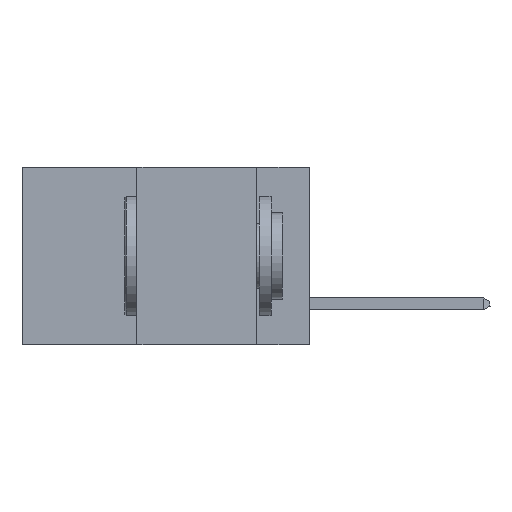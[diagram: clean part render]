
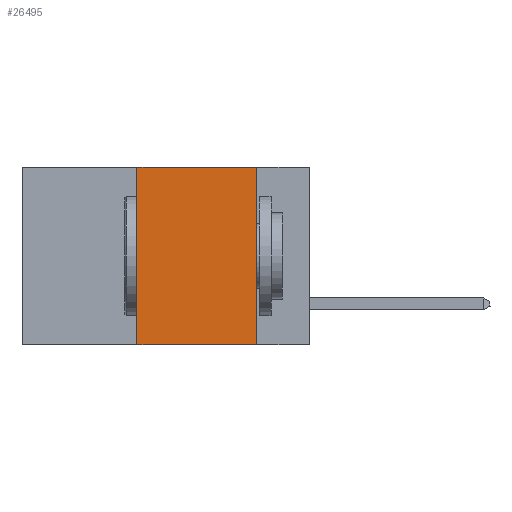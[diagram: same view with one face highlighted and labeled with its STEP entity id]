
A CAD part, left-side view. The second image highlights one B-rep face of the part: STEP entity #26495.
In plain terms, the highlighted planar face has unit normal (-1, 0, 0).
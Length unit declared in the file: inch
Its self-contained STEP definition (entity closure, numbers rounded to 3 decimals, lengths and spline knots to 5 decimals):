
#259 = EDGE_CURVE ( 'NONE', #32341, #35100, #21879, .T. ) ;
#385 = CARTESIAN_POINT ( 'NONE',  ( 0., 0.6, -0.37 ) ) ;
#1940 = AXIS2_PLACEMENT_3D ( 'NONE', #23389, #32214, #39652 ) ;
#6469 = VECTOR ( 'NONE', #30810, 39.37008 ) ;
#12043 = CARTESIAN_POINT ( 'NONE',  ( 0., 0.11, 0. ) ) ;
#13521 = CARTESIAN_POINT ( 'NONE',  ( 0., 0.6, 0. ) ) ;
#14008 = VECTOR ( 'NONE', #38672, 39.37008 ) ;
#15373 = VECTOR ( 'NONE', #23713, 39.37008 ) ;
#16250 = FACE_OUTER_BOUND ( 'NONE', #34864, .T. ) ;
#18440 = CARTESIAN_POINT ( 'NONE',  ( 0., 0.11, -0.37 ) ) ;
#19712 = CARTESIAN_POINT ( 'NONE',  ( 0., 0.36, 0. ) ) ;
#20656 = DIRECTION ( 'NONE',  ( 0., -1., 0. ) ) ;
#21879 = LINE ( 'NONE', #385, #6469 ) ;
#23027 = VECTOR ( 'NONE', #20656, 39.37008 ) ;
#23389 = CARTESIAN_POINT ( 'NONE',  ( 0., 0.6, 0. ) ) ;
#23713 = DIRECTION ( 'NONE',  ( 0., 0., -1. ) ) ;
#24348 = CARTESIAN_POINT ( 'NONE',  ( 0., 0.11, 0. ) ) ;
#24901 = CARTESIAN_POINT ( 'NONE',  ( 0., 0.36, -0.37 ) ) ;
#26495 = ADVANCED_FACE ( 'NONE', ( #16250 ), #35881, .F. ) ;
#27166 = ORIENTED_EDGE ( 'NONE', *, *, #259, .T. ) ;
#28327 = CARTESIAN_POINT ( 'NONE',  ( 0., 0.36, 0. ) ) ;
#30810 = DIRECTION ( 'NONE',  ( 0., -1., 0. ) ) ;
#32214 = DIRECTION ( 'NONE',  ( 1., 0., 0. ) ) ;
#32341 = VERTEX_POINT ( 'NONE', #24901 ) ;
#32445 = ORIENTED_EDGE ( 'NONE', *, *, #39499, .F. ) ;
#32481 = LINE ( 'NONE', #19712, #14008 ) ;
#34438 = EDGE_CURVE ( 'NONE', #32341, #36157, #32481, .T. ) ;
#34864 = EDGE_LOOP ( 'NONE', ( #32445, #36519, #47747, #27166 ) ) ;
#35100 = VERTEX_POINT ( 'NONE', #18440 ) ;
#35881 = PLANE ( 'NONE',  #1940 ) ;
#36157 = VERTEX_POINT ( 'NONE', #28327 ) ;
#36519 = ORIENTED_EDGE ( 'NONE', *, *, #43780, .F. ) ;
#38672 = DIRECTION ( 'NONE',  ( 0., 0., 1. ) ) ;
#39499 = EDGE_CURVE ( 'NONE', #43546, #35100, #46864, .T. ) ;
#39652 = DIRECTION ( 'NONE',  ( 0., 0., -1. ) ) ;
#43546 = VERTEX_POINT ( 'NONE', #12043 ) ;
#43780 = EDGE_CURVE ( 'NONE', #36157, #43546, #44420, .T. ) ;
#44420 = LINE ( 'NONE', #13521, #23027 ) ;
#46864 = LINE ( 'NONE', #24348, #15373 ) ;
#47747 = ORIENTED_EDGE ( 'NONE', *, *, #34438, .F. ) ;
